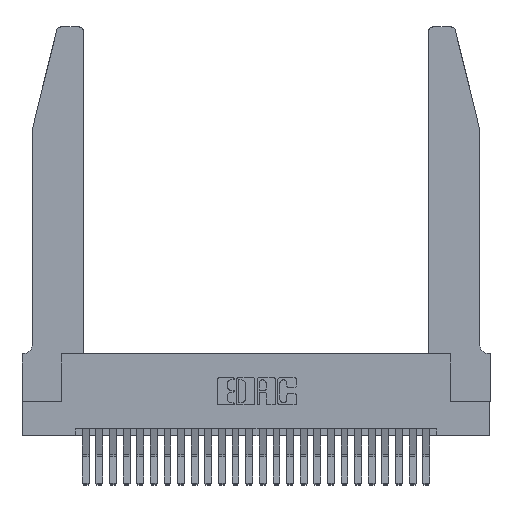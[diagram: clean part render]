
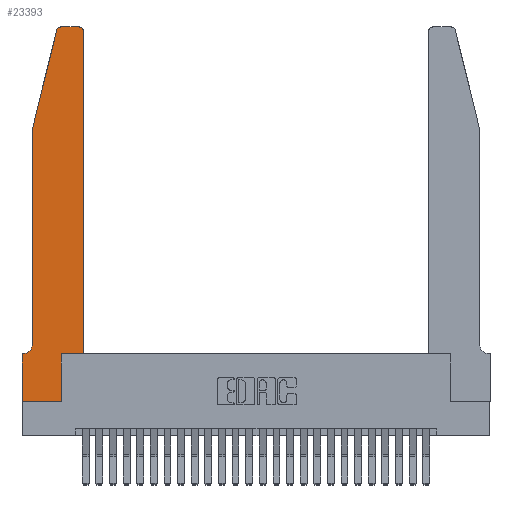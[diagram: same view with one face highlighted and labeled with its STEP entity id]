
A CAD part, top view. The second image highlights one B-rep face of the part: STEP entity #23393.
In plain terms, the highlighted planar face has unit normal (0, 0, 1).
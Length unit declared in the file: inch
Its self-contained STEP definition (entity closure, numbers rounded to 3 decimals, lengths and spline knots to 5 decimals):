
#733 = VERTEX_POINT ( 'NONE', #3979 ) ;
#805 = DIRECTION ( 'NONE',  ( 0., 0., -1. ) ) ;
#1058 = CARTESIAN_POINT ( 'NONE',  ( 0.2865, 0.35, 0.37 ) ) ;
#1143 = VERTEX_POINT ( 'NONE', #5929 ) ;
#1230 = LINE ( 'NONE', #7825, #9817 ) ;
#1262 = DIRECTION ( 'NONE',  ( 0., 1., 0. ) ) ;
#1520 = CARTESIAN_POINT ( 'NONE',  ( 0.4505, 0.35, 0.37 ) ) ;
#2010 = VECTOR ( 'NONE', #1262, 39.37008 ) ;
#2280 = VERTEX_POINT ( 'NONE', #10769 ) ;
#2347 = CARTESIAN_POINT ( 'NONE',  ( 0.0755, 2., 0.37 ) ) ;
#2454 = CARTESIAN_POINT ( 'NONE',  ( 0., 0., 0.37 ) ) ;
#2554 = DIRECTION ( 'NONE',  ( 1., 0., 0. ) ) ;
#3055 = CARTESIAN_POINT ( 'NONE',  ( 0.2865, 0., 0.37 ) ) ;
#3089 = CARTESIAN_POINT ( 'NONE',  ( 0.0055, 0.35, 0.37 ) ) ;
#3109 = DIRECTION ( 'NONE',  ( 0., -1., 0. ) ) ;
#3324 = DIRECTION ( 'NONE',  ( 1., 0., 0. ) ) ;
#3355 = LINE ( 'NONE', #1520, #2010 ) ;
#3979 = CARTESIAN_POINT ( 'NONE',  ( 0.284, 2.75, 0.37 ) ) ;
#4045 = EDGE_CURVE ( 'NONE', #25339, #12628, #19616, .T. ) ;
#4264 = ORIENTED_EDGE ( 'NONE', *, *, #26700, .T. ) ;
#4671 = ORIENTED_EDGE ( 'NONE', *, *, #21495, .T. ) ;
#4826 = DIRECTION ( 'NONE',  ( 0., -1., 0. ) ) ;
#5023 = EDGE_CURVE ( 'NONE', #733, #25107, #9571, .T. ) ;
#5569 = CARTESIAN_POINT ( 'NONE',  ( 0.25487, 2.72718, 0.37 ) ) ;
#5849 = EDGE_CURVE ( 'NONE', #19222, #2280, #13898, .T. ) ;
#5871 = DIRECTION ( 'NONE',  ( -1., 0., 0. ) ) ;
#5929 = CARTESIAN_POINT ( 'NONE',  ( 0.4505, 0.35, 0.37 ) ) ;
#5986 = VERTEX_POINT ( 'NONE', #2347 ) ;
#6244 = CARTESIAN_POINT ( 'NONE',  ( 0.0055, 0.42, 0.37 ) ) ;
#6284 = VECTOR ( 'NONE', #2554, 39.37008 ) ;
#6319 = CARTESIAN_POINT ( 'NONE',  ( 0.4205, 2.72, 0.37 ) ) ;
#6797 = CARTESIAN_POINT ( 'NONE',  ( 0., 0., 0.37 ) ) ;
#6916 = CIRCLE ( 'NONE', #17926, 0.07 ) ;
#7040 = LINE ( 'NONE', #21031, #10036 ) ;
#7093 = CARTESIAN_POINT ( 'NONE',  ( 0.0755, 0.42, 0.37 ) ) ;
#7161 = CARTESIAN_POINT ( 'NONE',  ( 0.4505, 0.35, 0.37 ) ) ;
#7214 = FACE_OUTER_BOUND ( 'NONE', #14071, .T. ) ;
#7627 = LINE ( 'NONE', #23650, #9939 ) ;
#7769 = ORIENTED_EDGE ( 'NONE', *, *, #5023, .T. ) ;
#7825 = CARTESIAN_POINT ( 'NONE',  ( 0.2865, 0.35, 0.37 ) ) ;
#8246 = VERTEX_POINT ( 'NONE', #1058 ) ;
#8261 = ORIENTED_EDGE ( 'NONE', *, *, #12640, .T. ) ;
#8455 = DIRECTION ( 'NONE',  ( 1., 0., 0. ) ) ;
#9259 = CARTESIAN_POINT ( 'NONE',  ( 0.4505, 2.72, 0.37 ) ) ;
#9381 = DIRECTION ( 'NONE',  ( -1., 0., 0. ) ) ;
#9559 = AXIS2_PLACEMENT_3D ( 'NONE', #17519, #11253, #19717 ) ;
#9571 = CIRCLE ( 'NONE', #12563, 0.03 ) ;
#9817 = VECTOR ( 'NONE', #14606, 39.37008 ) ;
#9939 = VECTOR ( 'NONE', #10885, 39.37008 ) ;
#10036 = VECTOR ( 'NONE', #5871, 39.37008 ) ;
#10769 = CARTESIAN_POINT ( 'NONE',  ( 0.4205, 2.75, 0.37 ) ) ;
#10885 = DIRECTION ( 'NONE',  ( -1., 0., 0. ) ) ;
#11253 = DIRECTION ( 'NONE',  ( 0., 0., 1. ) ) ;
#11888 = ORIENTED_EDGE ( 'NONE', *, *, #18093, .T. ) ;
#11907 = CARTESIAN_POINT ( 'NONE',  ( 0.0755, 2., 0.37 ) ) ;
#12403 = AXIS2_PLACEMENT_3D ( 'NONE', #6319, #12911, #8455 ) ;
#12563 = AXIS2_PLACEMENT_3D ( 'NONE', #16052, #22330, #3324 ) ;
#12628 = VERTEX_POINT ( 'NONE', #6797 ) ;
#12640 = EDGE_CURVE ( 'NONE', #8246, #1143, #22266, .T. ) ;
#12790 = EDGE_CURVE ( 'NONE', #1143, #19222, #3355, .T. ) ;
#12890 = ORIENTED_EDGE ( 'NONE', *, *, #4045, .T. ) ;
#12911 = DIRECTION ( 'NONE',  ( 0., 0., 1. ) ) ;
#13027 = CARTESIAN_POINT ( 'NONE',  ( 0., 0., 0.37 ) ) ;
#13898 = CIRCLE ( 'NONE', #12403, 0.03 ) ;
#13972 = VECTOR ( 'NONE', #3109, 39.37008 ) ;
#14004 = VERTEX_POINT ( 'NONE', #3055 ) ;
#14071 = EDGE_LOOP ( 'NONE', ( #15843, #7769, #26817, #11888, #4671, #24181, #12890, #4264, #15988, #8261, #14739, #26198 ) ) ;
#14595 = DIRECTION ( 'NONE',  ( -0.239, -0.971, 0. ) ) ;
#14606 = DIRECTION ( 'NONE',  ( 0., 1., 0. ) ) ;
#14739 = ORIENTED_EDGE ( 'NONE', *, *, #12790, .T. ) ;
#15259 = EDGE_CURVE ( 'NONE', #14004, #8246, #1230, .T. ) ;
#15594 = VERTEX_POINT ( 'NONE', #3089 ) ;
#15757 = LINE ( 'NONE', #11907, #20420 ) ;
#15843 = ORIENTED_EDGE ( 'NONE', *, *, #19557, .T. ) ;
#15988 = ORIENTED_EDGE ( 'NONE', *, *, #15259, .T. ) ;
#16052 = CARTESIAN_POINT ( 'NONE',  ( 0.284, 2.72, 0.37 ) ) ;
#17519 = CARTESIAN_POINT ( 'NONE',  ( 0., 0.35, 0.37 ) ) ;
#17926 = AXIS2_PLACEMENT_3D ( 'NONE', #6244, #805, #9381 ) ;
#18093 = EDGE_CURVE ( 'NONE', #5986, #19494, #21889, .T. ) ;
#18680 = EDGE_CURVE ( 'NONE', #25107, #5986, #15757, .T. ) ;
#19222 = VERTEX_POINT ( 'NONE', #9259 ) ;
#19494 = VERTEX_POINT ( 'NONE', #7093 ) ;
#19557 = EDGE_CURVE ( 'NONE', #2280, #733, #7040, .T. ) ;
#19616 = LINE ( 'NONE', #13027, #13972 ) ;
#19618 = VECTOR ( 'NONE', #19798, 39.37008 ) ;
#19717 = DIRECTION ( 'NONE',  ( 1., 0., 0. ) ) ;
#19798 = DIRECTION ( 'NONE',  ( 1., 0., 0. ) ) ;
#20420 = VECTOR ( 'NONE', #14595, 39.37008 ) ;
#21031 = CARTESIAN_POINT ( 'NONE',  ( 0.2605, 2.75, 0.37 ) ) ;
#21231 = VECTOR ( 'NONE', #4826, 39.37008 ) ;
#21495 = EDGE_CURVE ( 'NONE', #19494, #15594, #6916, .T. ) ;
#21889 = LINE ( 'NONE', #25756, #21231 ) ;
#22266 = LINE ( 'NONE', #7161, #19618 ) ;
#22330 = DIRECTION ( 'NONE',  ( 0., 0., 1. ) ) ;
#23393 = ADVANCED_FACE ( 'NONE', ( #7214 ), #23917, .T. ) ;
#23650 = CARTESIAN_POINT ( 'NONE',  ( 0.0755, 0.35, 0.37 ) ) ;
#23917 = PLANE ( 'NONE',  #9559 ) ;
#24181 = ORIENTED_EDGE ( 'NONE', *, *, #26724, .T. ) ;
#24515 = LINE ( 'NONE', #2454, #6284 ) ;
#25107 = VERTEX_POINT ( 'NONE', #5569 ) ;
#25339 = VERTEX_POINT ( 'NONE', #25549 ) ;
#25549 = CARTESIAN_POINT ( 'NONE',  ( 0., 0.35, 0.37 ) ) ;
#25756 = CARTESIAN_POINT ( 'NONE',  ( 0.0755, 2., 0.37 ) ) ;
#26198 = ORIENTED_EDGE ( 'NONE', *, *, #5849, .T. ) ;
#26700 = EDGE_CURVE ( 'NONE', #12628, #14004, #24515, .T. ) ;
#26724 = EDGE_CURVE ( 'NONE', #15594, #25339, #7627, .T. ) ;
#26817 = ORIENTED_EDGE ( 'NONE', *, *, #18680, .T. ) ;
